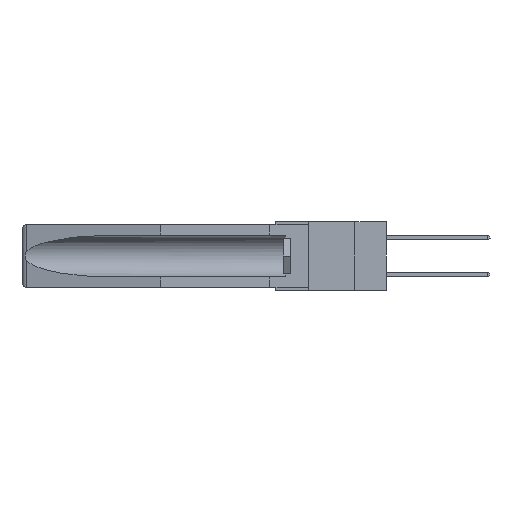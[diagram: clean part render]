
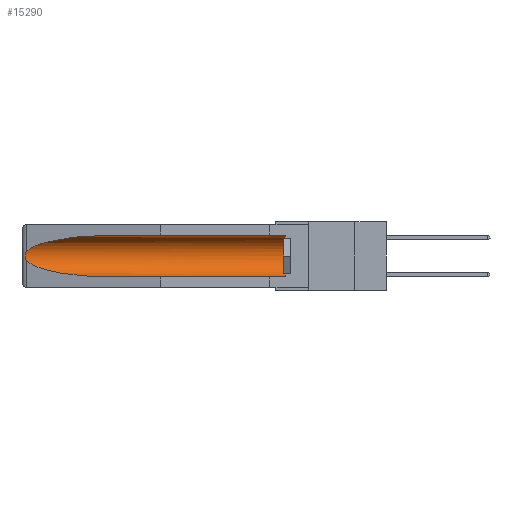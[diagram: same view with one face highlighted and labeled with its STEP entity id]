
A CAD part, left-side view. The second image highlights one B-rep face of the part: STEP entity #15290.
In plain terms, the highlighted cylindrical face has radius 2.857 mm (diameter 5.715 mm), a partial arc.
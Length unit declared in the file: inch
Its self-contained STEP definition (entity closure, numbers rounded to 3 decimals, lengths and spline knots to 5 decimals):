
#263 = CARTESIAN_POINT ( 'NONE',  ( 0.26537, 1.52718, -0.19328 ) ) ;
#1532 = ORIENTED_EDGE ( 'NONE', *, *, #4539, .T. ) ;
#1620 = AXIS2_PLACEMENT_3D ( 'NONE', #7005, #9110, #24178 ) ;
#1866 = CARTESIAN_POINT ( 'NONE',  ( 0.2673, 1.5327, -0.16383 ) ) ;
#2339 = CARTESIAN_POINT ( 'NONE',  ( 0.155, 1.07973, -0.059 ) ) ;
#2430 = EDGE_CURVE ( 'NONE', #13314, #19016, #22824, .T. ) ;
#2595 = EDGE_CURVE ( 'NONE', #4076, #9401, #23534, .T. ) ;
#3321 = EDGE_CURVE ( 'NONE', #17329, #4076, #23835, .T. ) ;
#3743 = ORIENTED_EDGE ( 'NONE', *, *, #3321, .T. ) ;
#4009 = CARTESIAN_POINT ( 'NONE',  ( 0.2673, 1.53269, -0.17917 ) ) ;
#4076 = VERTEX_POINT ( 'NONE', #2339 ) ;
#4080 = CARTESIAN_POINT ( 'NONE',  ( 0.26537, 1.52718, -0.14972 ) ) ;
#4088 = CARTESIAN_POINT ( 'NONE',  ( 0.155, -0.30754, -0.059 ) ) ;
#4271 = CARTESIAN_POINT ( 'NONE',  ( 0.21114, 1.30732, -0.059 ) ) ;
#4539 = EDGE_CURVE ( 'NONE', #9401, #13314, #25610, .T. ) ;
#5712 = CARTESIAN_POINT ( 'NONE',  ( 0.155, -0.30754, -0.1715 ) ) ;
#6230 = CARTESIAN_POINT ( 'NONE',  ( 0.26655, 1.53094, -0.18657 ) ) ;
#6868 = VECTOR ( 'NONE', #8506, 39.37008 ) ;
#7005 = CARTESIAN_POINT ( 'NONE',  ( 0.155, 0.126, -0.1715 ) ) ;
#7156 = EDGE_LOOP ( 'NONE', ( #9514, #1532, #13619, #8571, #12117, #3743 ) ) ;
#7175 = CIRCLE ( 'NONE', #1620, 0.1125 ) ;
#7515 = DIRECTION ( 'NONE',  ( 0., 1., 0. ) ) ;
#8506 = DIRECTION ( 'NONE',  ( 0., 1., 0. ) ) ;
#8571 = ORIENTED_EDGE ( 'NONE', *, *, #22671, .F. ) ;
#9110 = DIRECTION ( 'NONE',  ( 0., -1., 0. ) ) ;
#9401 = VERTEX_POINT ( 'NONE', #27395 ) ;
#9462 = EDGE_CURVE ( 'NONE', #22109, #17329, #7175, .T. ) ;
#9514 = ORIENTED_EDGE ( 'NONE', *, *, #2595, .T. ) ;
#10519 = CARTESIAN_POINT ( 'NONE',  ( 0.26537, 1.52718, -0.14972 ) ) ;
#10618 = CARTESIAN_POINT ( 'NONE',  ( 0.26537, 1.52718, -0.19328 ) ) ;
#10786 = CARTESIAN_POINT ( 'NONE',  ( 0.25451, 1.48313, -0.09465 ) ) ;
#11001 = VECTOR ( 'NONE', #7515, 39.37008 ) ;
#11914 = CARTESIAN_POINT ( 'NONE',  ( 0.155, 0.126, -0.284 ) ) ;
#12117 = ORIENTED_EDGE ( 'NONE', *, *, #9462, .T. ) ;
#13314 = VERTEX_POINT ( 'NONE', #263 ) ;
#13619 = ORIENTED_EDGE ( 'NONE', *, *, #2430, .T. ) ;
#14043 = CYLINDRICAL_SURFACE ( 'NONE', #24616, 0.1125 ) ;
#15076 = CARTESIAN_POINT ( 'NONE',  ( 0.155, 1.07973, -0.284 ) ) ;
#15290 = ADVANCED_FACE ( 'NONE', ( #15745 ), #14043, .F. ) ;
#15745 = FACE_OUTER_BOUND ( 'NONE', #7156, .T. ) ;
#17072 = CARTESIAN_POINT ( 'NONE',  ( 0.2675, 1.53308, -0.16763 ) ) ;
#17329 = VERTEX_POINT ( 'NONE', #20591 ) ;
#18127 = LINE ( 'NONE', #18342, #11001 ) ;
#18342 = CARTESIAN_POINT ( 'NONE',  ( 0.155, -0.30754, -0.284 ) ) ;
#19016 = VERTEX_POINT ( 'NONE', #15076 ) ;
#19236 = CARTESIAN_POINT ( 'NONE',  ( 0.2675, 1.53308, -0.17534 ) ) ;
#20297 = CARTESIAN_POINT ( 'NONE',  ( 0.26537, 1.52718, -0.19328 ) ) ;
#20591 = CARTESIAN_POINT ( 'NONE',  ( 0.155, 0.126, -0.059 ) ) ;
#21423 = CARTESIAN_POINT ( 'NONE',  ( 0.26597, 1.5296, -0.19026 ) ) ;
#22109 = VERTEX_POINT ( 'NONE', #11914 ) ;
#22281 = CARTESIAN_POINT ( 'NONE',  ( 0.155, 1.07973, -0.284 ) ) ;
#22671 = EDGE_CURVE ( 'NONE', #22109, #19016, #18127, .T. ) ;
#22824 =( BOUNDED_CURVE ( )  B_SPLINE_CURVE ( 3, ( #20297, #26705, #26893, #22281 ),
 .UNSPECIFIED., .F., .F. ) 
 B_SPLINE_CURVE_WITH_KNOTS ( ( 4, 4 ),
 ( 0.1948, 1.5708 ),
 .UNSPECIFIED. ) 
 CURVE ( )  GEOMETRIC_REPRESENTATION_ITEM ( )  RATIONAL_B_SPLINE_CURVE ( ( 1., 0.848, 0.848, 1. ) ) 
 REPRESENTATION_ITEM ( '' )  );
#23534 =( BOUNDED_CURVE ( )  B_SPLINE_CURVE ( 3, ( #26128, #4271, #10786, #4080 ),
 .UNSPECIFIED., .F., .T. ) 
 B_SPLINE_CURVE_WITH_KNOTS ( ( 4, 4 ),
 ( 4.71239, 6.08839 ),
 .UNSPECIFIED. ) 
 CURVE ( )  GEOMETRIC_REPRESENTATION_ITEM ( )  RATIONAL_B_SPLINE_CURVE ( ( 1., 0.848, 0.848, 1. ) ) 
 REPRESENTATION_ITEM ( '' )  );
#23835 = LINE ( 'NONE', #4088, #6868 ) ;
#24178 = DIRECTION ( 'NONE',  ( 0., 0., 1. ) ) ;
#24616 = AXIS2_PLACEMENT_3D ( 'NONE', #5712, #27438, #27253 ) ;
#25610 = B_SPLINE_CURVE_WITH_KNOTS ( 'NONE', 3,
 ( #10519, #25686, #27862, #1866, #17072, #19236, #4009, #6230, #21423, #10618 ),
 .UNSPECIFIED., .F., .F.,
 ( 4, 2, 2, 2, 4 ),
 ( 0., 0.00029, 0.00058, 0.00087, 0.00117 ),
 .UNSPECIFIED. ) ;
#25686 = CARTESIAN_POINT ( 'NONE',  ( 0.26597, 1.52961, -0.15275 ) ) ;
#26128 = CARTESIAN_POINT ( 'NONE',  ( 0.155, 1.07973, -0.059 ) ) ;
#26705 = CARTESIAN_POINT ( 'NONE',  ( 0.25451, 1.48313, -0.24835 ) ) ;
#26893 = CARTESIAN_POINT ( 'NONE',  ( 0.21114, 1.30732, -0.284 ) ) ;
#27253 = DIRECTION ( 'NONE',  ( 0., 0., 1. ) ) ;
#27395 = CARTESIAN_POINT ( 'NONE',  ( 0.26537, 1.52718, -0.14972 ) ) ;
#27438 = DIRECTION ( 'NONE',  ( 0., 1., 0. ) ) ;
#27862 = CARTESIAN_POINT ( 'NONE',  ( 0.26654, 1.53092, -0.15636 ) ) ;
